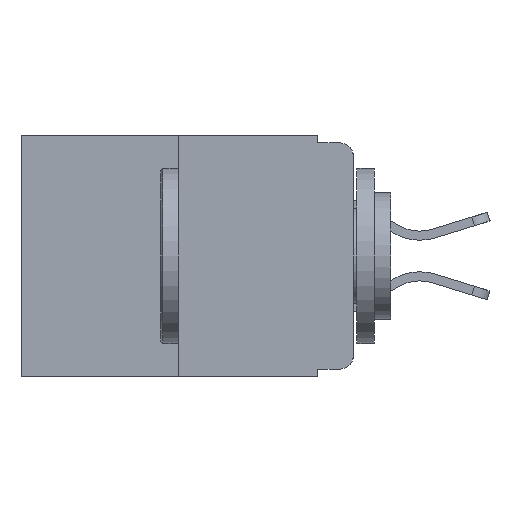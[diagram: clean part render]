
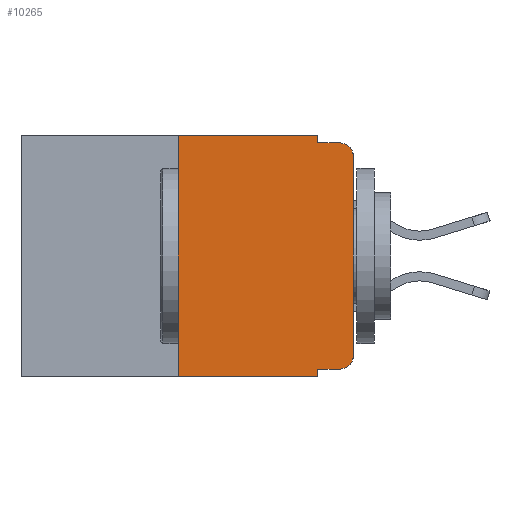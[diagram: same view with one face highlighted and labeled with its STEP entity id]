
A CAD part, left-side view. The second image highlights one B-rep face of the part: STEP entity #10265.
In plain terms, the highlighted planar face has unit normal (-1, 0, 0).
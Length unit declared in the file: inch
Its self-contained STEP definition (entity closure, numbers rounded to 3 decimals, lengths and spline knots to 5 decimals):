
#170 = ORIENTED_EDGE ( 'NONE', *, *, #13437, .F. ) ;
#174 = AXIS2_PLACEMENT_3D ( 'NONE', #5799, #3137, #12190 ) ;
#398 = AXIS2_PLACEMENT_3D ( 'NONE', #15824, #8400, #404 ) ;
#404 = DIRECTION ( 'NONE',  ( 0., 0., -1. ) ) ;
#474 = CARTESIAN_POINT ( 'NONE',  ( 0., 0.051, 0. ) ) ;
#530 = CARTESIAN_POINT ( 'NONE',  ( 0., 0.02, -0.333 ) ) ;
#899 = DIRECTION ( 'NONE',  ( 0., -1., 0. ) ) ;
#1026 = ORIENTED_EDGE ( 'NONE', *, *, #11886, .T. ) ;
#1179 = CARTESIAN_POINT ( 'NONE',  ( 0., 0.051, -0.333 ) ) ;
#1215 = VERTEX_POINT ( 'NONE', #1179 ) ;
#1466 = VECTOR ( 'NONE', #16384, 39.37008 ) ;
#1467 = ORIENTED_EDGE ( 'NONE', *, *, #11679, .T. ) ;
#1596 = CARTESIAN_POINT ( 'NONE',  ( 0., 0.25, 0. ) ) ;
#1755 = DIRECTION ( 'NONE',  ( 0., 0., -1. ) ) ;
#1903 = VERTEX_POINT ( 'NONE', #16618 ) ;
#2261 = ORIENTED_EDGE ( 'NONE', *, *, #4793, .T. ) ;
#2682 = VERTEX_POINT ( 'NONE', #5535 ) ;
#2968 = EDGE_CURVE ( 'NONE', #6686, #6074, #7280, .T. ) ;
#2975 = CARTESIAN_POINT ( 'NONE',  ( 0., 0.051, -0.01 ) ) ;
#3054 = DIRECTION ( 'NONE',  ( 0., 0., -1. ) ) ;
#3137 = DIRECTION ( 'NONE',  ( 1., 0., 0. ) ) ;
#3626 = CARTESIAN_POINT ( 'NONE',  ( 0., 0.473, -0.343 ) ) ;
#3630 = VERTEX_POINT ( 'NONE', #7324 ) ;
#4437 = FACE_OUTER_BOUND ( 'NONE', #12100, .T. ) ;
#4520 = CARTESIAN_POINT ( 'NONE',  ( 0., 0., 0. ) ) ;
#4793 = EDGE_CURVE ( 'NONE', #1215, #6686, #9428, .T. ) ;
#5072 = LINE ( 'NONE', #15163, #1466 ) ;
#5535 = CARTESIAN_POINT ( 'NONE',  ( 0., 0.02, -0.01 ) ) ;
#5613 = CARTESIAN_POINT ( 'NONE',  ( 0., 0.051, -0.333 ) ) ;
#5692 = EDGE_CURVE ( 'NONE', #1215, #1903, #5968, .T. ) ;
#5799 = CARTESIAN_POINT ( 'NONE',  ( 0., 0.473, 0. ) ) ;
#5865 = VECTOR ( 'NONE', #14613, 39.37008 ) ;
#5874 = DIRECTION ( 'NONE',  ( 0., 0., 1. ) ) ;
#5894 = ORIENTED_EDGE ( 'NONE', *, *, #2968, .T. ) ;
#5968 = LINE ( 'NONE', #8352, #12299 ) ;
#6051 = LINE ( 'NONE', #3626, #12379 ) ;
#6074 = VERTEX_POINT ( 'NONE', #10269 ) ;
#6093 = DIRECTION ( 'NONE',  ( 0., 0., 1. ) ) ;
#6686 = VERTEX_POINT ( 'NONE', #530 ) ;
#7280 = CIRCLE ( 'NONE', #15055, 0.02 ) ;
#7307 = VECTOR ( 'NONE', #6093, 39.37008 ) ;
#7324 = CARTESIAN_POINT ( 'NONE',  ( 0., 0., -0.03 ) ) ;
#7334 = ORIENTED_EDGE ( 'NONE', *, *, #7454, .F. ) ;
#7398 = CARTESIAN_POINT ( 'NONE',  ( 0., 0.25, 0. ) ) ;
#7454 = EDGE_CURVE ( 'NONE', #9589, #14756, #8113, .T. ) ;
#8113 = LINE ( 'NONE', #7398, #7307 ) ;
#8352 = CARTESIAN_POINT ( 'NONE',  ( 0., 0.051, 0. ) ) ;
#8400 = DIRECTION ( 'NONE',  ( -1., 0., 0. ) ) ;
#9168 = EDGE_CURVE ( 'NONE', #12221, #13388, #16027, .T. ) ;
#9284 = VECTOR ( 'NONE', #5874, 39.37008 ) ;
#9314 = LINE ( 'NONE', #9708, #5865 ) ;
#9428 = LINE ( 'NONE', #5613, #12717 ) ;
#9589 = VERTEX_POINT ( 'NONE', #13055 ) ;
#9708 = CARTESIAN_POINT ( 'NONE',  ( 0., 0.473, 0. ) ) ;
#9994 = EDGE_CURVE ( 'NONE', #13388, #2682, #5072, .T. ) ;
#10265 = ADVANCED_FACE ( 'NONE', ( #4437 ), #10936, .F. ) ;
#10269 = CARTESIAN_POINT ( 'NONE',  ( 0., 0., -0.313 ) ) ;
#10470 = DIRECTION ( 'NONE',  ( 0., -1., 0. ) ) ;
#10759 = CARTESIAN_POINT ( 'NONE',  ( 0., 0.051, 0. ) ) ;
#10824 = EDGE_CURVE ( 'NONE', #3630, #2682, #12606, .T. ) ;
#10936 = PLANE ( 'NONE',  #174 ) ;
#11679 = EDGE_CURVE ( 'NONE', #6074, #3630, #16606, .T. ) ;
#11874 = ORIENTED_EDGE ( 'NONE', *, *, #10824, .T. ) ;
#11886 = EDGE_CURVE ( 'NONE', #9589, #1903, #6051, .T. ) ;
#12100 = EDGE_LOOP ( 'NONE', ( #1467, #11874, #15698, #16460, #170, #7334, #1026, #15127, #2261, #5894 ) ) ;
#12190 = DIRECTION ( 'NONE',  ( 0., 0., -1. ) ) ;
#12221 = VERTEX_POINT ( 'NONE', #10759 ) ;
#12299 = VECTOR ( 'NONE', #3054, 39.37008 ) ;
#12379 = VECTOR ( 'NONE', #899, 39.37008 ) ;
#12606 = CIRCLE ( 'NONE', #398, 0.02 ) ;
#12717 = VECTOR ( 'NONE', #10470, 39.37008 ) ;
#13055 = CARTESIAN_POINT ( 'NONE',  ( 0., 0.25, -0.343 ) ) ;
#13388 = VERTEX_POINT ( 'NONE', #2975 ) ;
#13437 = EDGE_CURVE ( 'NONE', #14756, #12221, #9314, .T. ) ;
#13728 = DIRECTION ( 'NONE',  ( 0., 0., -1. ) ) ;
#14613 = DIRECTION ( 'NONE',  ( 0., -1., 0. ) ) ;
#14756 = VERTEX_POINT ( 'NONE', #1596 ) ;
#15055 = AXIS2_PLACEMENT_3D ( 'NONE', #15436, #15351, #13728 ) ;
#15127 = ORIENTED_EDGE ( 'NONE', *, *, #5692, .F. ) ;
#15163 = CARTESIAN_POINT ( 'NONE',  ( 0., 0.051, -0.01 ) ) ;
#15351 = DIRECTION ( 'NONE',  ( -1., 0., 0. ) ) ;
#15436 = CARTESIAN_POINT ( 'NONE',  ( 0., 0.02, -0.313 ) ) ;
#15698 = ORIENTED_EDGE ( 'NONE', *, *, #9994, .F. ) ;
#15824 = CARTESIAN_POINT ( 'NONE',  ( 0., 0.02, -0.03 ) ) ;
#16027 = LINE ( 'NONE', #474, #16411 ) ;
#16384 = DIRECTION ( 'NONE',  ( 0., -1., 0. ) ) ;
#16411 = VECTOR ( 'NONE', #1755, 39.37008 ) ;
#16460 = ORIENTED_EDGE ( 'NONE', *, *, #9168, .F. ) ;
#16606 = LINE ( 'NONE', #4520, #9284 ) ;
#16618 = CARTESIAN_POINT ( 'NONE',  ( 0., 0.051, -0.343 ) ) ;
